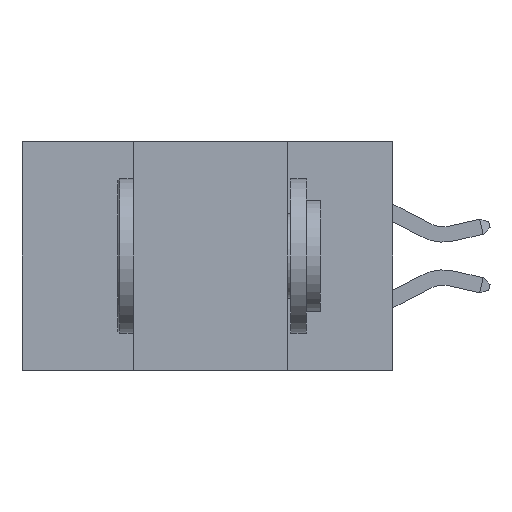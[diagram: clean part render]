
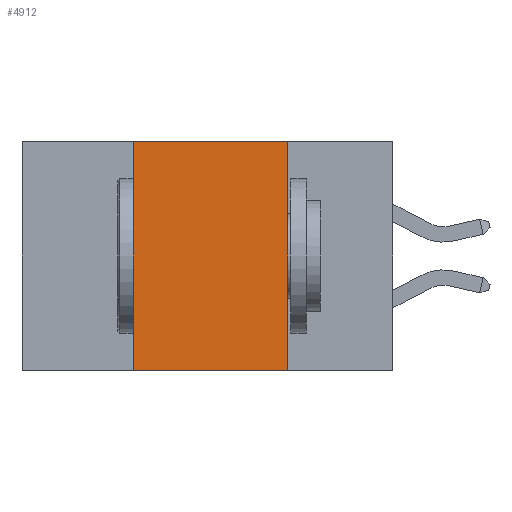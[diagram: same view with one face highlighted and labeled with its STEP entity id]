
A CAD part, left-side view. The second image highlights one B-rep face of the part: STEP entity #4912.
In plain terms, the highlighted planar face has unit normal (-1, 0, 0).
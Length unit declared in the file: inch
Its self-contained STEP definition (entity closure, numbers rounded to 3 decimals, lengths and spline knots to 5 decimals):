
#402 = CARTESIAN_POINT ( 'NONE',  ( 0., 0.6, 0. ) ) ;
#481 = ORIENTED_EDGE ( 'NONE', *, *, #2507, .F. ) ;
#700 = LINE ( 'NONE', #402, #8595 ) ;
#777 = EDGE_CURVE ( 'NONE', #4116, #5065, #9278, .T. ) ;
#1630 = CARTESIAN_POINT ( 'NONE',  ( 0., 0.17, 0. ) ) ;
#1998 = CARTESIAN_POINT ( 'NONE',  ( 0., 0.17, 0. ) ) ;
#2132 = CARTESIAN_POINT ( 'NONE',  ( 0., 0.42, 0. ) ) ;
#2206 = CARTESIAN_POINT ( 'NONE',  ( 0., 0.42, -0.37 ) ) ;
#2507 = EDGE_CURVE ( 'NONE', #5065, #11587, #700, .T. ) ;
#2582 = LINE ( 'NONE', #8954, #13617 ) ;
#3542 = DIRECTION ( 'NONE',  ( 0., -1., 0. ) ) ;
#4116 = VERTEX_POINT ( 'NONE', #2206 ) ;
#4196 = DIRECTION ( 'NONE',  ( 1., 0., 0. ) ) ;
#4402 = EDGE_LOOP ( 'NONE', ( #9851, #481, #7058, #13340 ) ) ;
#4912 = ADVANCED_FACE ( 'NONE', ( #7204 ), #8624, .F. ) ;
#5065 = VERTEX_POINT ( 'NONE', #11293 ) ;
#5125 = LINE ( 'NONE', #1630, #12790 ) ;
#5920 = VERTEX_POINT ( 'NONE', #13818 ) ;
#6436 = EDGE_CURVE ( 'NONE', #11587, #5920, #5125, .T. ) ;
#7058 = ORIENTED_EDGE ( 'NONE', *, *, #777, .F. ) ;
#7204 = FACE_OUTER_BOUND ( 'NONE', #4402, .T. ) ;
#7570 = CARTESIAN_POINT ( 'NONE',  ( 0., 0.6, 0. ) ) ;
#8272 = VECTOR ( 'NONE', #8472, 39.37008 ) ;
#8399 = AXIS2_PLACEMENT_3D ( 'NONE', #7570, #4196, #9660 ) ;
#8472 = DIRECTION ( 'NONE',  ( 0., 0., 1. ) ) ;
#8595 = VECTOR ( 'NONE', #12171, 39.37008 ) ;
#8624 = PLANE ( 'NONE',  #8399 ) ;
#8954 = CARTESIAN_POINT ( 'NONE',  ( 0., 0.6, -0.37 ) ) ;
#9278 = LINE ( 'NONE', #2132, #8272 ) ;
#9660 = DIRECTION ( 'NONE',  ( 0., 0., -1. ) ) ;
#9851 = ORIENTED_EDGE ( 'NONE', *, *, #6436, .F. ) ;
#11293 = CARTESIAN_POINT ( 'NONE',  ( 0., 0.42, 0. ) ) ;
#11587 = VERTEX_POINT ( 'NONE', #1998 ) ;
#12171 = DIRECTION ( 'NONE',  ( 0., -1., 0. ) ) ;
#12219 = DIRECTION ( 'NONE',  ( 0., 0., -1. ) ) ;
#12790 = VECTOR ( 'NONE', #12219, 39.37008 ) ;
#13216 = EDGE_CURVE ( 'NONE', #4116, #5920, #2582, .T. ) ;
#13340 = ORIENTED_EDGE ( 'NONE', *, *, #13216, .T. ) ;
#13617 = VECTOR ( 'NONE', #3542, 39.37008 ) ;
#13818 = CARTESIAN_POINT ( 'NONE',  ( 0., 0.17, -0.37 ) ) ;
